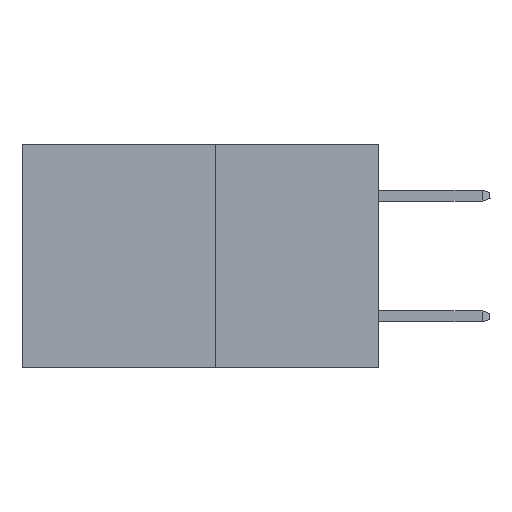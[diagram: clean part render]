
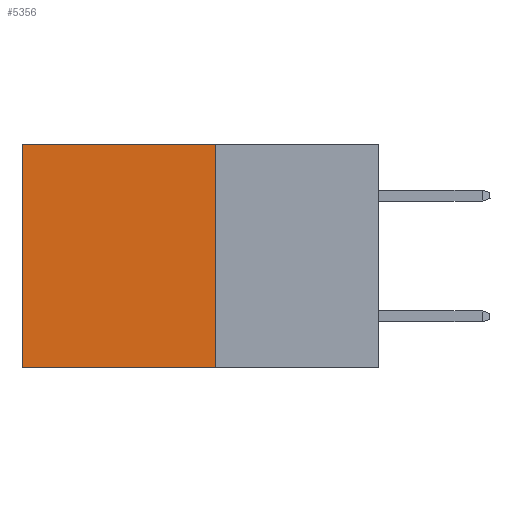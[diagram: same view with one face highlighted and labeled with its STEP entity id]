
A CAD part, left-side view. The second image highlights one B-rep face of the part: STEP entity #5356.
In plain terms, the highlighted planar face has unit normal (-1, 0, 0).
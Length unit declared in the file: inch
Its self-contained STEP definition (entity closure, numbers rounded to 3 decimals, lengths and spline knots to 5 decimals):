
#3413 = CARTESIAN_POINT ( 'NONE',  ( 0.277, 0.59, -0.37 ) ) ;
#4906 = EDGE_LOOP ( 'NONE', ( #7060, #9891, #23831, #23458 ) ) ;
#5331 = DIRECTION ( 'NONE',  ( 0., 1., 0. ) ) ;
#5356 = ADVANCED_FACE ( 'NONE', ( #30063 ), #15006, .F. ) ;
#7060 = ORIENTED_EDGE ( 'NONE', *, *, #24063, .T. ) ;
#8063 = VECTOR ( 'NONE', #24079, 39.37008 ) ;
#9891 = ORIENTED_EDGE ( 'NONE', *, *, #10306, .F. ) ;
#10306 = EDGE_CURVE ( 'NONE', #29709, #21125, #10429, .T. ) ;
#10429 = LINE ( 'NONE', #20795, #28992 ) ;
#11441 = CARTESIAN_POINT ( 'NONE',  ( 0.277, 0.27, 0. ) ) ;
#11593 = EDGE_CURVE ( 'NONE', #32973, #29709, #26555, .T. ) ;
#13122 = CARTESIAN_POINT ( 'NONE',  ( 0.277, 0.27, -0.37 ) ) ;
#13144 = DIRECTION ( 'NONE',  ( 0., 0., -1. ) ) ;
#13814 = CARTESIAN_POINT ( 'NONE',  ( 0.277, 0.59, 0. ) ) ;
#13936 = VECTOR ( 'NONE', #20818, 39.37008 ) ;
#14153 = DIRECTION ( 'NONE',  ( 1., 0., 0. ) ) ;
#14988 = LINE ( 'NONE', #11441, #8063 ) ;
#15006 = PLANE ( 'NONE',  #32498 ) ;
#15953 = CARTESIAN_POINT ( 'NONE',  ( 0.277, 0.27, -0.37 ) ) ;
#16676 = DIRECTION ( 'NONE',  ( 0., 0., -1. ) ) ;
#17861 = VECTOR ( 'NONE', #16676, 39.37008 ) ;
#20177 = CARTESIAN_POINT ( 'NONE',  ( 0.277, 0.27, 0. ) ) ;
#20795 = CARTESIAN_POINT ( 'NONE',  ( 0.277, 0.27, -0.37 ) ) ;
#20818 = DIRECTION ( 'NONE',  ( 0., 0., -1. ) ) ;
#21125 = VERTEX_POINT ( 'NONE', #24962 ) ;
#23024 = VERTEX_POINT ( 'NONE', #13814 ) ;
#23458 = ORIENTED_EDGE ( 'NONE', *, *, #25430, .T. ) ;
#23831 = ORIENTED_EDGE ( 'NONE', *, *, #11593, .F. ) ;
#24063 = EDGE_CURVE ( 'NONE', #23024, #21125, #31930, .T. ) ;
#24079 = DIRECTION ( 'NONE',  ( 0., 1., 0. ) ) ;
#24962 = CARTESIAN_POINT ( 'NONE',  ( 0.277, 0.59, -0.37 ) ) ;
#25430 = EDGE_CURVE ( 'NONE', #32973, #23024, #14988, .T. ) ;
#26555 = LINE ( 'NONE', #13122, #13936 ) ;
#28992 = VECTOR ( 'NONE', #5331, 39.37008 ) ;
#29709 = VERTEX_POINT ( 'NONE', #30305 ) ;
#30063 = FACE_OUTER_BOUND ( 'NONE', #4906, .T. ) ;
#30305 = CARTESIAN_POINT ( 'NONE',  ( 0.277, 0.27, -0.37 ) ) ;
#31930 = LINE ( 'NONE', #3413, #17861 ) ;
#32498 = AXIS2_PLACEMENT_3D ( 'NONE', #15953, #14153, #13144 ) ;
#32973 = VERTEX_POINT ( 'NONE', #20177 ) ;
